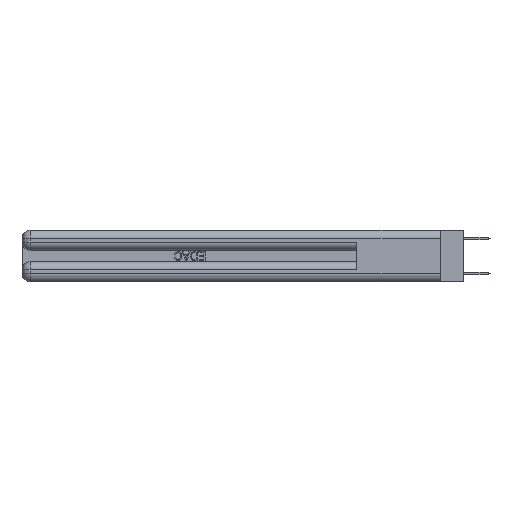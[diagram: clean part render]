
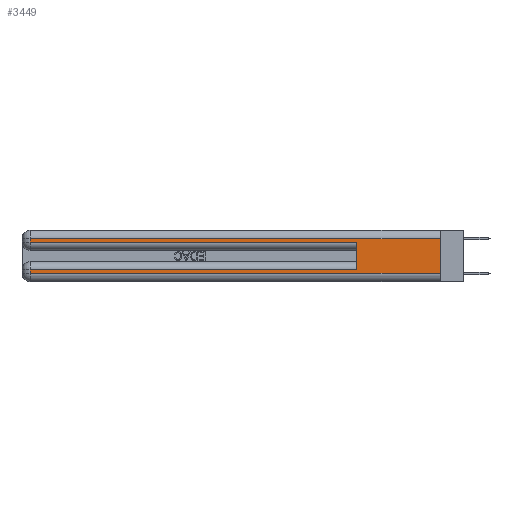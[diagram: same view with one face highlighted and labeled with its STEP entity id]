
A CAD part, left-side view. The second image highlights one B-rep face of the part: STEP entity #3449.
In plain terms, the highlighted planar face has unit normal (-1, 0, 0).
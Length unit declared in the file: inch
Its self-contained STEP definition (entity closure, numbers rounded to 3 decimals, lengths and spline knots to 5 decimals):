
#566 = VECTOR ( 'NONE', #20128, 39.37008 ) ;
#1086 = VERTEX_POINT ( 'NONE', #12522 ) ;
#1324 = VECTOR ( 'NONE', #25710, 39.37008 ) ;
#2610 = CARTESIAN_POINT ( 'NONE',  ( 0., 0., 0.37 ) ) ;
#3449 = ADVANCED_FACE ( 'NONE', ( #14019 ), #17621, .F. ) ;
#3977 = AXIS2_PLACEMENT_3D ( 'NONE', #17768, #17618, #17576 ) ;
#4346 = CARTESIAN_POINT ( 'NONE',  ( 0., 2.94, 0.31 ) ) ;
#5228 = DIRECTION ( 'NONE',  ( 0., 0., -1. ) ) ;
#5740 = VERTEX_POINT ( 'NONE', #4346 ) ;
#7121 = CARTESIAN_POINT ( 'NONE',  ( 0., 2.94, 0.37 ) ) ;
#7216 = VERTEX_POINT ( 'NONE', #10294 ) ;
#7409 = DIRECTION ( 'NONE',  ( 0., 1., 0. ) ) ;
#7921 = VERTEX_POINT ( 'NONE', #11870 ) ;
#9067 = LINE ( 'NONE', #23229, #1324 ) ;
#9504 = EDGE_CURVE ( 'NONE', #23615, #11353, #32797, .T. ) ;
#10206 = EDGE_CURVE ( 'NONE', #21597, #1086, #14015, .T. ) ;
#10294 = CARTESIAN_POINT ( 'NONE',  ( 0., 2.94, 0.06 ) ) ;
#11353 = VERTEX_POINT ( 'NONE', #15828 ) ;
#11731 = DIRECTION ( 'NONE',  ( 0., 0., -1. ) ) ;
#11870 = CARTESIAN_POINT ( 'NONE',  ( 0., 2.94, 0.085 ) ) ;
#12059 = VECTOR ( 'NONE', #12889, 39.37008 ) ;
#12522 = CARTESIAN_POINT ( 'NONE',  ( 0., 0., 0.06 ) ) ;
#12889 = DIRECTION ( 'NONE',  ( 0., -1., 0. ) ) ;
#13215 = VECTOR ( 'NONE', #5228, 39.37008 ) ;
#14015 = LINE ( 'NONE', #2610, #13215 ) ;
#14019 = FACE_OUTER_BOUND ( 'NONE', #21658, .T. ) ;
#15439 = DIRECTION ( 'NONE',  ( 0., -1., 0. ) ) ;
#15828 = CARTESIAN_POINT ( 'NONE',  ( 0., 0.6, 0.285 ) ) ;
#17070 = CARTESIAN_POINT ( 'NONE',  ( 0., 2.94, 0.285 ) ) ;
#17576 = DIRECTION ( 'NONE',  ( 0., 0., -1. ) ) ;
#17618 = DIRECTION ( 'NONE',  ( 1., 0., 0. ) ) ;
#17621 = PLANE ( 'NONE',  #3977 ) ;
#17768 = CARTESIAN_POINT ( 'NONE',  ( 0., 0., 0.37 ) ) ;
#18478 = EDGE_CURVE ( 'NONE', #7216, #1086, #21717, .T. ) ;
#18525 = CARTESIAN_POINT ( 'NONE',  ( 0., 0., 0.31 ) ) ;
#19008 = LINE ( 'NONE', #27715, #24921 ) ;
#19733 = ORIENTED_EDGE ( 'NONE', *, *, #10206, .F. ) ;
#20128 = DIRECTION ( 'NONE',  ( 0., 1., 0. ) ) ;
#20132 = VECTOR ( 'NONE', #15439, 39.37008 ) ;
#20148 = ORIENTED_EDGE ( 'NONE', *, *, #24481, .T. ) ;
#20686 = ORIENTED_EDGE ( 'NONE', *, *, #24235, .T. ) ;
#21026 = ORIENTED_EDGE ( 'NONE', *, *, #9504, .T. ) ;
#21597 = VERTEX_POINT ( 'NONE', #18525 ) ;
#21614 = CARTESIAN_POINT ( 'NONE',  ( 0., 0.6, 0.085 ) ) ;
#21658 = EDGE_LOOP ( 'NONE', ( #19733, #20148, #20686, #21026, #27680, #22588, #24130, #27228 ) ) ;
#21717 = LINE ( 'NONE', #22953, #20132 ) ;
#22588 = ORIENTED_EDGE ( 'NONE', *, *, #25656, .T. ) ;
#22953 = CARTESIAN_POINT ( 'NONE',  ( 0., 0., 0.06 ) ) ;
#23229 = CARTESIAN_POINT ( 'NONE',  ( 0., 0.6, 0.145 ) ) ;
#23615 = VERTEX_POINT ( 'NONE', #17070 ) ;
#24018 = VERTEX_POINT ( 'NONE', #21614 ) ;
#24130 = ORIENTED_EDGE ( 'NONE', *, *, #25246, .T. ) ;
#24235 = EDGE_CURVE ( 'NONE', #5740, #23615, #27189, .T. ) ;
#24428 = EDGE_CURVE ( 'NONE', #24018, #11353, #9067, .T. ) ;
#24481 = EDGE_CURVE ( 'NONE', #21597, #5740, #27754, .T. ) ;
#24921 = VECTOR ( 'NONE', #7409, 39.37008 ) ;
#25246 = EDGE_CURVE ( 'NONE', #7921, #7216, #29952, .T. ) ;
#25656 = EDGE_CURVE ( 'NONE', #24018, #7921, #19008, .T. ) ;
#25710 = DIRECTION ( 'NONE',  ( 0., 0., 1. ) ) ;
#26840 = CARTESIAN_POINT ( 'NONE',  ( 0., 2.94, 0.37 ) ) ;
#27189 = LINE ( 'NONE', #7121, #32193 ) ;
#27228 = ORIENTED_EDGE ( 'NONE', *, *, #18478, .T. ) ;
#27680 = ORIENTED_EDGE ( 'NONE', *, *, #24428, .F. ) ;
#27715 = CARTESIAN_POINT ( 'NONE',  ( 0., 0., 0.085 ) ) ;
#27754 = LINE ( 'NONE', #32454, #566 ) ;
#27958 = CARTESIAN_POINT ( 'NONE',  ( 0., 0., 0.285 ) ) ;
#29952 = LINE ( 'NONE', #26840, #31483 ) ;
#31483 = VECTOR ( 'NONE', #11731, 39.37008 ) ;
#32193 = VECTOR ( 'NONE', #32286, 39.37008 ) ;
#32286 = DIRECTION ( 'NONE',  ( 0., 0., -1. ) ) ;
#32454 = CARTESIAN_POINT ( 'NONE',  ( 0., 0., 0.31 ) ) ;
#32797 = LINE ( 'NONE', #27958, #12059 ) ;
